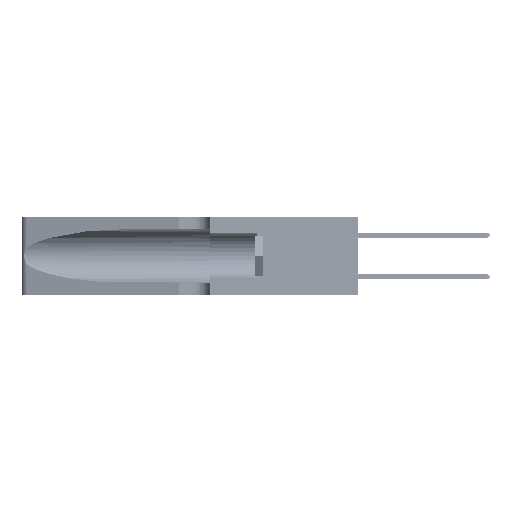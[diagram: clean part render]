
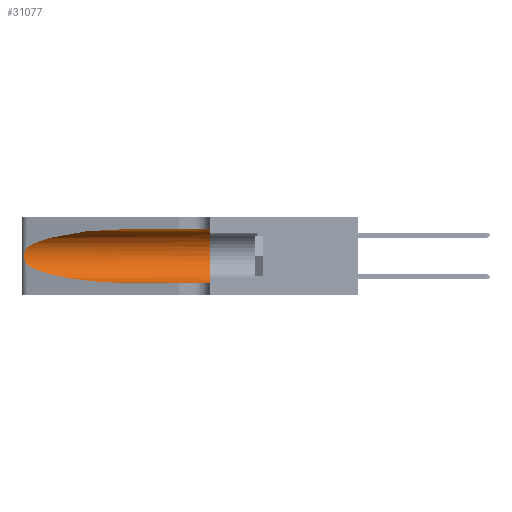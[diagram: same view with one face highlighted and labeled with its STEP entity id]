
A CAD part, left-side view. The second image highlights one B-rep face of the part: STEP entity #31077.
In plain terms, the highlighted cylindrical face has radius 3.308 mm (diameter 6.617 mm), a partial arc.
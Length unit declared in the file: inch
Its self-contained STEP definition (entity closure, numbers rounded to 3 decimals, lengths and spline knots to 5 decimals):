
#473 = VERTEX_POINT ( 'NONE', #24483 ) ;
#889 = CARTESIAN_POINT ( 'NONE',  ( 0.25555, 1.22994, 0.2215 ) ) ;
#1246 = CARTESIAN_POINT ( 'NONE',  ( 0.26075, 1.23896, 0.178 ) ) ;
#2007 = CYLINDRICAL_SURFACE ( 'NONE', #47126, 0.13025 ) ;
#3308 = CARTESIAN_POINT ( 'NONE',  ( 0.1305, 0.72297, 0.05475 ) ) ;
#3568 = EDGE_CURVE ( 'NONE', #44931, #47974, #28702, .T. ) ;
#5272 = CARTESIAN_POINT ( 'NONE',  ( 0.25856, 1.23593, 0.16098 ) ) ;
#5509 = VERTEX_POINT ( 'NONE', #14067 ) ;
#6062 = EDGE_LOOP ( 'NONE', ( #9390, #37246, #50853, #46908, #10610, #32719 ) ) ;
#7445 = CARTESIAN_POINT ( 'NONE',  ( 0.2373, 1.15595, 0.08982 ) ) ;
#7567 = CARTESIAN_POINT ( 'NONE',  ( 0.1305, 0.35, 0.05475 ) ) ;
#7781 = CARTESIAN_POINT ( 'NONE',  ( 0.25487, 1.22718, 0.22369 ) ) ;
#8921 =( BOUNDED_CURVE ( )  B_SPLINE_CURVE ( 3, ( #51045, #7445, #39330, #15528 ),
 .UNSPECIFIED., .F., .F. ) 
 B_SPLINE_CURVE_WITH_KNOTS ( ( 4, 4 ),
 ( 3.44316, 4.71239 ),
 .UNSPECIFIED. ) 
 CURVE ( )  GEOMETRIC_REPRESENTATION_ITEM ( )  RATIONAL_B_SPLINE_CURVE ( ( 1., 0.87, 0.87, 1. ) ) 
 REPRESENTATION_ITEM ( '' )  );
#9323 = CARTESIAN_POINT ( 'NONE',  ( 0.25639, 1.23186, 0.15144 ) ) ;
#9390 = ORIENTED_EDGE ( 'NONE', *, *, #28032, .T. ) ;
#9723 = EDGE_CURVE ( 'NONE', #15051, #47974, #31047, .T. ) ;
#10074 = CARTESIAN_POINT ( 'NONE',  ( 0.1305, 1.61858, 0.31525 ) ) ;
#10198 = EDGE_CURVE ( 'NONE', #28908, #44931, #49502, .T. ) ;
#10610 = ORIENTED_EDGE ( 'NONE', *, *, #3568, .F. ) ;
#12640 = EDGE_CURVE ( 'NONE', #473, #5509, #27523, .T. ) ;
#13341 = CARTESIAN_POINT ( 'NONE',  ( 0.25487, 1.22718, 0.14631 ) ) ;
#14067 = CARTESIAN_POINT ( 'NONE',  ( 0.25487, 1.22718, 0.14631 ) ) ;
#14969 = DIRECTION ( 'NONE',  ( 0., 1., 0. ) ) ;
#15051 = VERTEX_POINT ( 'NONE', #3308 ) ;
#15528 = CARTESIAN_POINT ( 'NONE',  ( 0.1305, 0.72297, 0.05475 ) ) ;
#16550 = EDGE_CURVE ( 'NONE', #5509, #15051, #8921, .T. ) ;
#17229 = CARTESIAN_POINT ( 'NONE',  ( 0.25639, 1.23184, 0.21858 ) ) ;
#21239 = CARTESIAN_POINT ( 'NONE',  ( 0.25854, 1.2359, 0.20912 ) ) ;
#22149 = DIRECTION ( 'NONE',  ( 0., -1., 0. ) ) ;
#23617 = CARTESIAN_POINT ( 'NONE',  ( 0.1305, 0.35, 0.31525 ) ) ;
#23746 = CARTESIAN_POINT ( 'NONE',  ( 0.18966, 0.96281, 0.31525 ) ) ;
#24483 = CARTESIAN_POINT ( 'NONE',  ( 0.25487, 1.22718, 0.22369 ) ) ;
#25237 = CARTESIAN_POINT ( 'NONE',  ( 0.26075, 1.23896, 0.19203 ) ) ;
#27360 = DIRECTION ( 'NONE',  ( 0., 0., -1. ) ) ;
#27523 = B_SPLINE_CURVE_WITH_KNOTS ( 'NONE', 3,
 ( #33069, #889, #17229, #44977, #21239, #48910, #25237, #1246, #29223, #5272, #33231, #9323, #37202, #13341 ),
 .UNSPECIFIED., .F., .F.,
 ( 4, 2, 2, 2, 2, 2, 4 ),
 ( 0., 0.00027, 0.00053, 0.00107, 0.0016, 0.00187, 0.00214 ),
 .UNSPECIFIED. ) ;
#27799 = CARTESIAN_POINT ( 'NONE',  ( 0.1305, 1.61858, 0.05475 ) ) ;
#28032 = EDGE_CURVE ( 'NONE', #28908, #473, #32920, .T. ) ;
#28702 = CIRCLE ( 'NONE', #37665, 0.13025 ) ;
#28908 = VERTEX_POINT ( 'NONE', #49631 ) ;
#29223 = CARTESIAN_POINT ( 'NONE',  ( 0.26017, 1.23833, 0.17102 ) ) ;
#31047 = LINE ( 'NONE', #27799, #40328 ) ;
#31077 = ADVANCED_FACE ( 'NONE', ( #35173 ), #2007, .F. ) ;
#31726 = CARTESIAN_POINT ( 'NONE',  ( 0.2373, 1.15595, 0.28018 ) ) ;
#31795 = DIRECTION ( 'NONE',  ( 0., -1., 0. ) ) ;
#32719 = ORIENTED_EDGE ( 'NONE', *, *, #10198, .F. ) ;
#32920 =( BOUNDED_CURVE ( )  B_SPLINE_CURVE ( 3, ( #51390, #23746, #31726, #7781 ),
 .UNSPECIFIED., .F., .F. ) 
 B_SPLINE_CURVE_WITH_KNOTS ( ( 4, 4 ),
 ( 1.5708, 2.84003 ),
 .UNSPECIFIED. ) 
 CURVE ( )  GEOMETRIC_REPRESENTATION_ITEM ( )  RATIONAL_B_SPLINE_CURVE ( ( 1., 0.87, 0.87, 1. ) ) 
 REPRESENTATION_ITEM ( '' )  );
#33069 = CARTESIAN_POINT ( 'NONE',  ( 0.25487, 1.22718, 0.22369 ) ) ;
#33231 = CARTESIAN_POINT ( 'NONE',  ( 0.25789, 1.23486, 0.15765 ) ) ;
#35173 = FACE_OUTER_BOUND ( 'NONE', #6062, .T. ) ;
#37202 = CARTESIAN_POINT ( 'NONE',  ( 0.25555, 1.22993, 0.14849 ) ) ;
#37246 = ORIENTED_EDGE ( 'NONE', *, *, #12640, .T. ) ;
#37665 = AXIS2_PLACEMENT_3D ( 'NONE', #38807, #14969, #42770 ) ;
#38807 = CARTESIAN_POINT ( 'NONE',  ( 0.1305, 0.35, 0.185 ) ) ;
#39330 = CARTESIAN_POINT ( 'NONE',  ( 0.18966, 0.96281, 0.05475 ) ) ;
#40328 = VECTOR ( 'NONE', #31795, 39.37008 ) ;
#42770 = DIRECTION ( 'NONE',  ( 0., 0., 1. ) ) ;
#44931 = VERTEX_POINT ( 'NONE', #23617 ) ;
#44977 = CARTESIAN_POINT ( 'NONE',  ( 0.25787, 1.23484, 0.2124 ) ) ;
#46908 = ORIENTED_EDGE ( 'NONE', *, *, #9723, .T. ) ;
#47126 = AXIS2_PLACEMENT_3D ( 'NONE', #51183, #47228, #27360 ) ;
#47228 = DIRECTION ( 'NONE',  ( 0., -1., 0. ) ) ;
#47974 = VERTEX_POINT ( 'NONE', #7567 ) ;
#48276 = VECTOR ( 'NONE', #22149, 39.37008 ) ;
#48910 = CARTESIAN_POINT ( 'NONE',  ( 0.26018, 1.23835, 0.19895 ) ) ;
#49502 = LINE ( 'NONE', #10074, #48276 ) ;
#49631 = CARTESIAN_POINT ( 'NONE',  ( 0.1305, 0.72297, 0.31525 ) ) ;
#50853 = ORIENTED_EDGE ( 'NONE', *, *, #16550, .T. ) ;
#51045 = CARTESIAN_POINT ( 'NONE',  ( 0.25487, 1.22718, 0.14631 ) ) ;
#51183 = CARTESIAN_POINT ( 'NONE',  ( 0.1305, 1.61858, 0.185 ) ) ;
#51390 = CARTESIAN_POINT ( 'NONE',  ( 0.1305, 0.72297, 0.31525 ) ) ;
